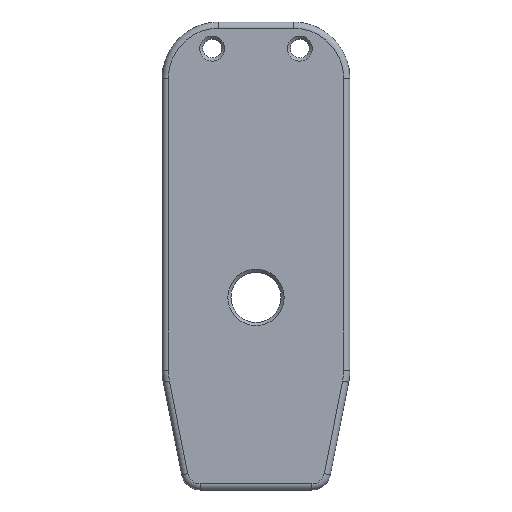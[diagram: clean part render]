
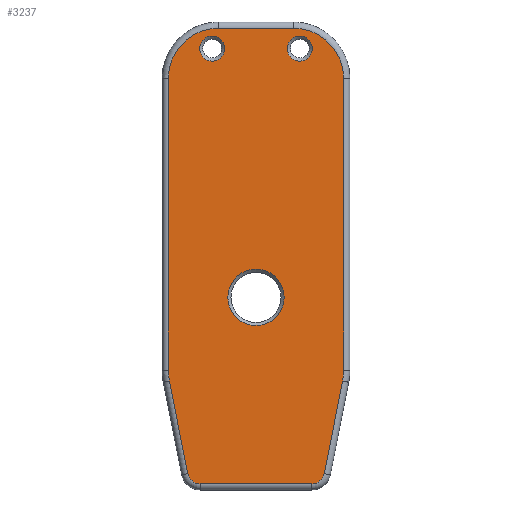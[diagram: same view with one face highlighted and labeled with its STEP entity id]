
A CAD part, front view. The second image highlights one B-rep face of the part: STEP entity #3237.
In plain terms, the highlighted planar face has unit normal (0, -1, 0).
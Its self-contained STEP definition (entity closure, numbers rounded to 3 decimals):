
#19=FACE_BOUND('',#1026,.T.);
#20=FACE_BOUND('',#1027,.T.);
#21=FACE_BOUND('',#1028,.T.);
#63=PLANE('',#3645);
#278=LINE('',#5805,#501);
#279=LINE('',#5816,#502);
#281=LINE('',#5828,#504);
#283=LINE('',#5840,#506);
#285=LINE('',#5852,#508);
#287=LINE('',#5864,#510);
#501=VECTOR('',#4488,10.);
#502=VECTOR('',#4501,10.);
#504=VECTOR('',#4515,10.);
#506=VECTOR('',#4529,10.);
#508=VECTOR('',#4543,10.);
#510=VECTOR('',#4557,10.);
#805=FACE_OUTER_BOUND('',#1025,.T.);
#1025=EDGE_LOOP('',(#2720,#2721,#2722,#2723,#2724,#2725,#2726,#2727,#2728,
#2729,#2730,#2731));
#1026=EDGE_LOOP('',(#2732));
#1027=EDGE_LOOP('',(#2733));
#1028=EDGE_LOOP('',(#2734));
#1283=CIRCLE('',#3605,8.);
#1287=CIRCLE('',#3611,9.);
#1291=CIRCLE('',#3617,2.);
#1295=CIRCLE('',#3623,2.);
#1299=CIRCLE('',#3629,9.);
#1302=CIRCLE('',#3634,8.);
#1307=CIRCLE('',#3646,4.5);
#1308=CIRCLE('',#3647,2.);
#1309=CIRCLE('',#3648,2.);
#1580=VERTEX_POINT('',#5798);
#1583=VERTEX_POINT('',#5803);
#1585=VERTEX_POINT('',#5808);
#1587=VERTEX_POINT('',#5814);
#1589=VERTEX_POINT('',#5820);
#1591=VERTEX_POINT('',#5826);
#1593=VERTEX_POINT('',#5832);
#1595=VERTEX_POINT('',#5838);
#1597=VERTEX_POINT('',#5844);
#1599=VERTEX_POINT('',#5850);
#1601=VERTEX_POINT('',#5856);
#1603=VERTEX_POINT('',#5862);
#1612=VERTEX_POINT('',#5899);
#1613=VERTEX_POINT('',#5901);
#1614=VERTEX_POINT('',#5903);
#1966=EDGE_CURVE('',#1583,#1580,#278,.T.);
#1968=EDGE_CURVE('',#1585,#1583,#1283,.T.);
#1971=EDGE_CURVE('',#1587,#1585,#279,.T.);
#1974=EDGE_CURVE('',#1589,#1587,#1287,.T.);
#1977=EDGE_CURVE('',#1591,#1589,#281,.T.);
#1980=EDGE_CURVE('',#1593,#1591,#1291,.T.);
#1983=EDGE_CURVE('',#1595,#1593,#283,.T.);
#1986=EDGE_CURVE('',#1597,#1595,#1295,.T.);
#1989=EDGE_CURVE('',#1599,#1597,#285,.T.);
#1992=EDGE_CURVE('',#1601,#1599,#1299,.T.);
#1995=EDGE_CURVE('',#1603,#1601,#287,.T.);
#1997=EDGE_CURVE('',#1580,#1603,#1302,.T.);
#2014=EDGE_CURVE('',#1612,#1612,#1307,.T.);
#2015=EDGE_CURVE('',#1613,#1613,#1308,.T.);
#2016=EDGE_CURVE('',#1614,#1614,#1309,.T.);
#2720=ORIENTED_EDGE('',*,*,#1966,.F.);
#2721=ORIENTED_EDGE('',*,*,#1968,.F.);
#2722=ORIENTED_EDGE('',*,*,#1971,.F.);
#2723=ORIENTED_EDGE('',*,*,#1974,.F.);
#2724=ORIENTED_EDGE('',*,*,#1977,.F.);
#2725=ORIENTED_EDGE('',*,*,#1980,.F.);
#2726=ORIENTED_EDGE('',*,*,#1983,.F.);
#2727=ORIENTED_EDGE('',*,*,#1986,.F.);
#2728=ORIENTED_EDGE('',*,*,#1989,.F.);
#2729=ORIENTED_EDGE('',*,*,#1992,.F.);
#2730=ORIENTED_EDGE('',*,*,#1995,.F.);
#2731=ORIENTED_EDGE('',*,*,#1997,.F.);
#2732=ORIENTED_EDGE('',*,*,#2014,.F.);
#2733=ORIENTED_EDGE('',*,*,#2015,.F.);
#2734=ORIENTED_EDGE('',*,*,#2016,.F.);
#3237=ADVANCED_FACE('',(#805,#19,#20,#21),#63,.T.);
#3605=AXIS2_PLACEMENT_3D('',#5810,#4493,#4494);
#3611=AXIS2_PLACEMENT_3D('',#5822,#4507,#4508);
#3617=AXIS2_PLACEMENT_3D('',#5834,#4521,#4522);
#3623=AXIS2_PLACEMENT_3D('',#5846,#4535,#4536);
#3629=AXIS2_PLACEMENT_3D('',#5858,#4549,#4550);
#3634=AXIS2_PLACEMENT_3D('',#5867,#4561,#4562);
#3645=AXIS2_PLACEMENT_3D('',#5898,#4595,#4596);
#3646=AXIS2_PLACEMENT_3D('',#5900,#4597,#4598);
#3647=AXIS2_PLACEMENT_3D('',#5902,#4599,#4600);
#3648=AXIS2_PLACEMENT_3D('',#5904,#4601,#4602);
#4488=DIRECTION('',(1.,0.,0.));
#4493=DIRECTION('center_axis',(0.,1.,0.));
#4494=DIRECTION('ref_axis',(-0.707,0.,0.707));
#4501=DIRECTION('',(0.,0.,1.));
#4507=DIRECTION('center_axis',(0.,1.,0.));
#4508=DIRECTION('ref_axis',(-0.995,0.,-0.097));
#4515=DIRECTION('',(-0.194,0.,0.981));
#4521=DIRECTION('center_axis',(0.,1.,0.));
#4522=DIRECTION('ref_axis',(-0.635,0.,-0.773));
#4529=DIRECTION('',(-1.,0.,0.));
#4535=DIRECTION('center_axis',(0.,1.,0.));
#4536=DIRECTION('ref_axis',(0.635,0.,-0.773));
#4543=DIRECTION('',(-0.194,0.,-0.981));
#4549=DIRECTION('center_axis',(0.,1.,0.));
#4550=DIRECTION('ref_axis',(0.995,0.,-0.097));
#4557=DIRECTION('',(0.,0.,-1.));
#4561=DIRECTION('center_axis',(0.,1.,0.));
#4562=DIRECTION('ref_axis',(0.707,0.,0.707));
#4595=DIRECTION('center_axis',(0.,-1.,0.));
#4596=DIRECTION('ref_axis',(1.,0.,0.));
#4597=DIRECTION('center_axis',(0.,-1.,0.));
#4598=DIRECTION('ref_axis',(-1.,0.,0.));
#4599=DIRECTION('center_axis',(0.,-1.,0.));
#4600=DIRECTION('ref_axis',(1.,0.,0.));
#4601=DIRECTION('center_axis',(0.,-1.,0.));
#4602=DIRECTION('ref_axis',(1.,0.,0.));
#5798=CARTESIAN_POINT('',(6.,17.5,29.5));
#5803=CARTESIAN_POINT('',(-6.,17.5,29.5));
#5805=CARTESIAN_POINT('',(-3.,17.5,29.5));
#5808=CARTESIAN_POINT('',(-14.,17.5,21.5));
#5810=CARTESIAN_POINT('Origin',(-6.,17.5,21.5));
#5814=CARTESIAN_POINT('',(-14.,17.5,-25.12));
#5816=CARTESIAN_POINT('',(-14.,17.5,-16.493));
#5820=CARTESIAN_POINT('',(-13.83,17.5,-26.863));
#5822=CARTESIAN_POINT('Origin',(-5.,17.5,-25.12));
#5826=CARTESIAN_POINT('',(-10.907,17.5,-41.664));
#5828=CARTESIAN_POINT('',(-14.007,17.5,-25.965));
#5832=CARTESIAN_POINT('',(-8.945,17.5,-43.277));
#5834=CARTESIAN_POINT('Origin',(-8.945,17.5,-41.277));
#5838=CARTESIAN_POINT('',(8.945,17.5,-43.277));
#5840=CARTESIAN_POINT('',(4.472,17.5,-43.277));
#5844=CARTESIAN_POINT('',(10.907,17.5,-41.664));
#5846=CARTESIAN_POINT('Origin',(8.945,17.5,-41.277));
#5850=CARTESIAN_POINT('',(13.83,17.5,-26.863));
#5852=CARTESIAN_POINT('',(15.563,17.5,-18.085));
#5856=CARTESIAN_POINT('',(14.,17.5,-25.12));
#5858=CARTESIAN_POINT('Origin',(5.,17.5,-25.12));
#5862=CARTESIAN_POINT('',(14.,17.5,21.5));
#5864=CARTESIAN_POINT('',(14.,17.5,7.306));
#5867=CARTESIAN_POINT('Origin',(6.,17.5,21.5));
#5898=CARTESIAN_POINT('Origin',(0.,17.5,-6.888));
#5899=CARTESIAN_POINT('',(4.5,17.5,-13.5));
#5900=CARTESIAN_POINT('Origin',(0.,17.5,-13.5));
#5901=CARTESIAN_POINT('',(-9.,17.5,26.25));
#5902=CARTESIAN_POINT('Origin',(-7.,17.5,26.25));
#5903=CARTESIAN_POINT('',(5.,17.5,26.25));
#5904=CARTESIAN_POINT('Origin',(7.,17.5,26.25));
